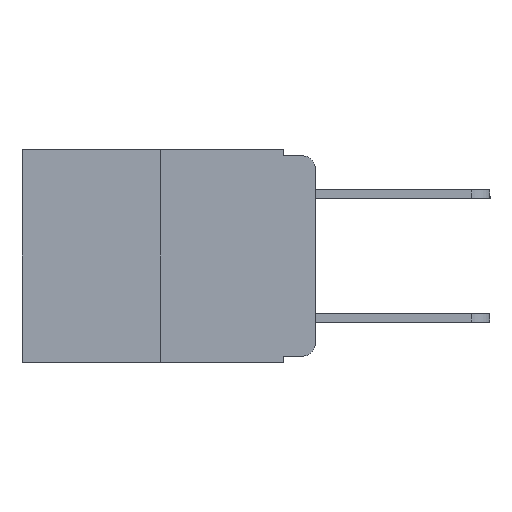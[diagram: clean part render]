
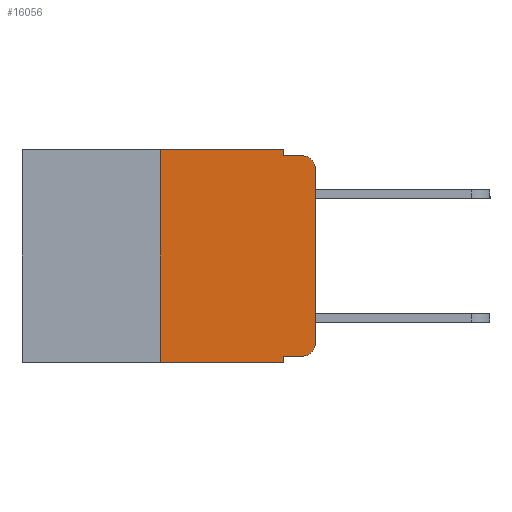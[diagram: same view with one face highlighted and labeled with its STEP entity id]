
A CAD part, left-side view. The second image highlights one B-rep face of the part: STEP entity #16056.
In plain terms, the highlighted planar face has unit normal (-1, 0, 0).
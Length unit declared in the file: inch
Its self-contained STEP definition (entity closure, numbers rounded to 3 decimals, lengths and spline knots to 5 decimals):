
#655 = AXIS2_PLACEMENT_3D ( 'NONE', #11144, #19857, #19832 ) ;
#678 = DIRECTION ( 'NONE',  ( 0., -1., 0. ) ) ;
#820 = PLANE ( 'NONE',  #15410 ) ;
#1188 = EDGE_CURVE ( 'NONE', #20459, #9759, #12174, .T. ) ;
#1946 = ORIENTED_EDGE ( 'NONE', *, *, #14422, .T. ) ;
#1962 = FACE_OUTER_BOUND ( 'NONE', #14310, .T. ) ;
#2280 = EDGE_CURVE ( 'NONE', #11897, #20130, #6315, .T. ) ;
#3038 = CIRCLE ( 'NONE', #655, 0.02 ) ;
#3355 = VECTOR ( 'NONE', #10498, 39.37008 ) ;
#3624 = VECTOR ( 'NONE', #18893, 39.37008 ) ;
#4244 = CARTESIAN_POINT ( 'NONE',  ( 0., 0.051, -0.333 ) ) ;
#4285 = CARTESIAN_POINT ( 'NONE',  ( 0., 0.051, -0.343 ) ) ;
#4413 = DIRECTION ( 'NONE',  ( 0., 0., -1. ) ) ;
#4495 = DIRECTION ( 'NONE',  ( -1., 0., 0. ) ) ;
#4949 = CARTESIAN_POINT ( 'NONE',  ( 0., 0.051, 0. ) ) ;
#5039 = VERTEX_POINT ( 'NONE', #12644 ) ;
#5262 = ORIENTED_EDGE ( 'NONE', *, *, #6532, .T. ) ;
#5283 = ORIENTED_EDGE ( 'NONE', *, *, #13573, .F. ) ;
#5623 = ORIENTED_EDGE ( 'NONE', *, *, #15453, .F. ) ;
#5785 = CARTESIAN_POINT ( 'NONE',  ( 0., 0.051, -0.01 ) ) ;
#5881 = CARTESIAN_POINT ( 'NONE',  ( 0., 0.25, 0. ) ) ;
#5952 = CARTESIAN_POINT ( 'NONE',  ( 0., 0.051, -0.333 ) ) ;
#6031 = VERTEX_POINT ( 'NONE', #21178 ) ;
#6315 = LINE ( 'NONE', #4949, #19304 ) ;
#6414 = ORIENTED_EDGE ( 'NONE', *, *, #10960, .F. ) ;
#6532 = EDGE_CURVE ( 'NONE', #11744, #6945, #3038, .T. ) ;
#6769 = ORIENTED_EDGE ( 'NONE', *, *, #1188, .F. ) ;
#6945 = VERTEX_POINT ( 'NONE', #8996 ) ;
#6985 = ORIENTED_EDGE ( 'NONE', *, *, #15138, .T. ) ;
#7006 = ORIENTED_EDGE ( 'NONE', *, *, #2280, .F. ) ;
#7128 = LINE ( 'NONE', #11366, #19098 ) ;
#7209 = DIRECTION ( 'NONE',  ( 0., 0., -1. ) ) ;
#7590 = CIRCLE ( 'NONE', #19342, 0.02 ) ;
#7690 = VECTOR ( 'NONE', #16742, 39.37008 ) ;
#7841 = VECTOR ( 'NONE', #16931, 39.37008 ) ;
#7929 = ORIENTED_EDGE ( 'NONE', *, *, #11879, .T. ) ;
#7950 = CARTESIAN_POINT ( 'NONE',  ( 0., 0.051, -0.01 ) ) ;
#8380 = VECTOR ( 'NONE', #12533, 39.37008 ) ;
#8388 = ORIENTED_EDGE ( 'NONE', *, *, #12528, .T. ) ;
#8996 = CARTESIAN_POINT ( 'NONE',  ( 0., 0.02, -0.01 ) ) ;
#9759 = VERTEX_POINT ( 'NONE', #5881 ) ;
#10395 = CARTESIAN_POINT ( 'NONE',  ( 0., 0., -0.313 ) ) ;
#10498 = DIRECTION ( 'NONE',  ( 0., 0., -1. ) ) ;
#10945 = CARTESIAN_POINT ( 'NONE',  ( 0., 0.473, -0.343 ) ) ;
#10960 = EDGE_CURVE ( 'NONE', #9759, #6031, #7128, .T. ) ;
#11144 = CARTESIAN_POINT ( 'NONE',  ( 0., 0.02, -0.03 ) ) ;
#11366 = CARTESIAN_POINT ( 'NONE',  ( 0., 0.473, 0. ) ) ;
#11744 = VERTEX_POINT ( 'NONE', #18601 ) ;
#11869 = VECTOR ( 'NONE', #678, 39.37008 ) ;
#11879 = EDGE_CURVE ( 'NONE', #11897, #5039, #12345, .T. ) ;
#11897 = VERTEX_POINT ( 'NONE', #5952 ) ;
#12174 = LINE ( 'NONE', #12727, #7690 ) ;
#12345 = LINE ( 'NONE', #4244, #11869 ) ;
#12528 = EDGE_CURVE ( 'NONE', #5039, #19828, #7590, .T. ) ;
#12533 = DIRECTION ( 'NONE',  ( 0., -1., 0. ) ) ;
#12644 = CARTESIAN_POINT ( 'NONE',  ( 0., 0.02, -0.333 ) ) ;
#12727 = CARTESIAN_POINT ( 'NONE',  ( 0., 0.25, 0. ) ) ;
#13573 = EDGE_CURVE ( 'NONE', #17481, #6945, #21123, .T. ) ;
#13696 = CARTESIAN_POINT ( 'NONE',  ( 0., 0., 0. ) ) ;
#14310 = EDGE_LOOP ( 'NONE', ( #1946, #5262, #5283, #5623, #6414, #6769, #6985, #7006, #7929, #8388 ) ) ;
#14409 = DIRECTION ( 'NONE',  ( 1., 0., 0. ) ) ;
#14422 = EDGE_CURVE ( 'NONE', #19828, #11744, #20097, .T. ) ;
#14494 = CARTESIAN_POINT ( 'NONE',  ( 0., 0.02, -0.313 ) ) ;
#15088 = LINE ( 'NONE', #19904, #3355 ) ;
#15138 = EDGE_CURVE ( 'NONE', #20459, #20130, #17022, .T. ) ;
#15410 = AXIS2_PLACEMENT_3D ( 'NONE', #15939, #14409, #4413 ) ;
#15453 = EDGE_CURVE ( 'NONE', #6031, #17481, #15088, .T. ) ;
#15939 = CARTESIAN_POINT ( 'NONE',  ( 0., 0.473, 0. ) ) ;
#16056 = ADVANCED_FACE ( 'NONE', ( #1962 ), #820, .F. ) ;
#16095 = DIRECTION ( 'NONE',  ( 0., 0., -1. ) ) ;
#16742 = DIRECTION ( 'NONE',  ( 0., 0., 1. ) ) ;
#16931 = DIRECTION ( 'NONE',  ( 0., 0., 1. ) ) ;
#17022 = LINE ( 'NONE', #10945, #8380 ) ;
#17481 = VERTEX_POINT ( 'NONE', #7950 ) ;
#18601 = CARTESIAN_POINT ( 'NONE',  ( 0., 0., -0.03 ) ) ;
#18893 = DIRECTION ( 'NONE',  ( 0., -1., 0. ) ) ;
#19098 = VECTOR ( 'NONE', #19252, 39.37008 ) ;
#19252 = DIRECTION ( 'NONE',  ( 0., -1., 0. ) ) ;
#19304 = VECTOR ( 'NONE', #7209, 39.37008 ) ;
#19342 = AXIS2_PLACEMENT_3D ( 'NONE', #14494, #4495, #16095 ) ;
#19828 = VERTEX_POINT ( 'NONE', #10395 ) ;
#19832 = DIRECTION ( 'NONE',  ( 0., 0., -1. ) ) ;
#19857 = DIRECTION ( 'NONE',  ( -1., 0., 0. ) ) ;
#19904 = CARTESIAN_POINT ( 'NONE',  ( 0., 0.051, 0. ) ) ;
#20097 = LINE ( 'NONE', #13696, #7841 ) ;
#20130 = VERTEX_POINT ( 'NONE', #4285 ) ;
#20459 = VERTEX_POINT ( 'NONE', #21151 ) ;
#21123 = LINE ( 'NONE', #5785, #3624 ) ;
#21151 = CARTESIAN_POINT ( 'NONE',  ( 0., 0.25, -0.343 ) ) ;
#21178 = CARTESIAN_POINT ( 'NONE',  ( 0., 0.051, 0. ) ) ;
